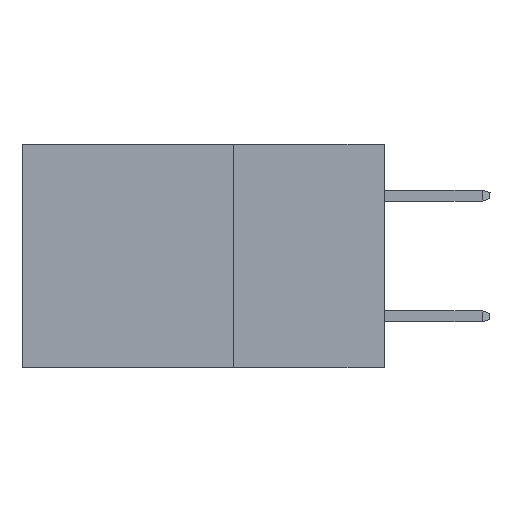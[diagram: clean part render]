
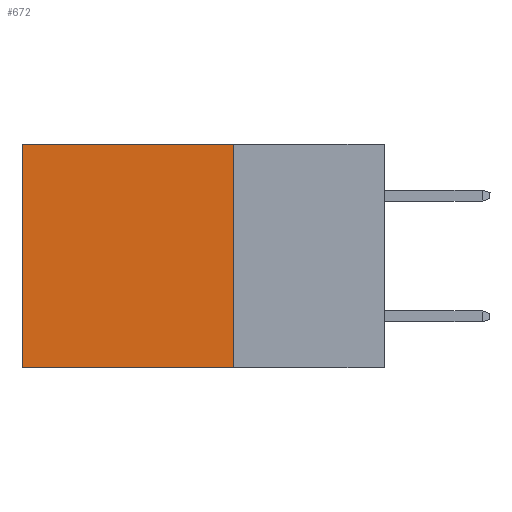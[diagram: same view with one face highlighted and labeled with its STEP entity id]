
A CAD part, left-side view. The second image highlights one B-rep face of the part: STEP entity #672.
In plain terms, the highlighted planar face has unit normal (-1, 0, 0).
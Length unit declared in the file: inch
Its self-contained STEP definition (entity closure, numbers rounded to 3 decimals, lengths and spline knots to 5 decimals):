
#672 = ADVANCED_FACE ( 'NONE', ( #2167 ), #1390, .F. ) ;
#751 = ORIENTED_EDGE ( 'NONE', *, *, #10423, .F. ) ;
#904 = CARTESIAN_POINT ( 'NONE',  ( 0.298, 0.6, 0. ) ) ;
#1065 = CARTESIAN_POINT ( 'NONE',  ( 0.298, 0.6, 0. ) ) ;
#1092 = ORIENTED_EDGE ( 'NONE', *, *, #1553, .F. ) ;
#1360 = LINE ( 'NONE', #7998, #1813 ) ;
#1390 = PLANE ( 'NONE',  #4530 ) ;
#1408 = DIRECTION ( 'NONE',  ( 0., 1., 0. ) ) ;
#1553 = EDGE_CURVE ( 'NONE', #9499, #7437, #1999, .T. ) ;
#1813 = VECTOR ( 'NONE', #3385, 39.37008 ) ;
#1849 = CARTESIAN_POINT ( 'NONE',  ( 0.298, 0.25, 0. ) ) ;
#1999 = LINE ( 'NONE', #6921, #11102 ) ;
#2167 = FACE_OUTER_BOUND ( 'NONE', #8779, .T. ) ;
#2579 = VECTOR ( 'NONE', #4663, 39.37008 ) ;
#3385 = DIRECTION ( 'NONE',  ( 0., 0., -1. ) ) ;
#3850 = LINE ( 'NONE', #904, #8636 ) ;
#4530 = AXIS2_PLACEMENT_3D ( 'NONE', #6015, #6788, #7035 ) ;
#4585 = EDGE_CURVE ( 'NONE', #6712, #10845, #6578, .T. ) ;
#4663 = DIRECTION ( 'NONE',  ( 0., 1., 0. ) ) ;
#5018 = ORIENTED_EDGE ( 'NONE', *, *, #9315, .T. ) ;
#5598 = CARTESIAN_POINT ( 'NONE',  ( 0.298, 0.25, -0.37 ) ) ;
#6015 = CARTESIAN_POINT ( 'NONE',  ( 0.298, 0.25, 0. ) ) ;
#6381 = DIRECTION ( 'NONE',  ( 0., 0., -1. ) ) ;
#6578 = LINE ( 'NONE', #8092, #2579 ) ;
#6712 = VERTEX_POINT ( 'NONE', #1849 ) ;
#6788 = DIRECTION ( 'NONE',  ( 1., 0., 0. ) ) ;
#6921 = CARTESIAN_POINT ( 'NONE',  ( 0.298, 0.25, -0.37 ) ) ;
#7035 = DIRECTION ( 'NONE',  ( 0., 0., -1. ) ) ;
#7437 = VERTEX_POINT ( 'NONE', #8575 ) ;
#7998 = CARTESIAN_POINT ( 'NONE',  ( 0.298, 0.25, 0. ) ) ;
#8092 = CARTESIAN_POINT ( 'NONE',  ( 0.298, 0.25, 0. ) ) ;
#8575 = CARTESIAN_POINT ( 'NONE',  ( 0.298, 0.6, -0.37 ) ) ;
#8636 = VECTOR ( 'NONE', #6381, 39.37008 ) ;
#8779 = EDGE_LOOP ( 'NONE', ( #5018, #1092, #751, #11189 ) ) ;
#9315 = EDGE_CURVE ( 'NONE', #10845, #7437, #3850, .T. ) ;
#9499 = VERTEX_POINT ( 'NONE', #5598 ) ;
#10423 = EDGE_CURVE ( 'NONE', #6712, #9499, #1360, .T. ) ;
#10845 = VERTEX_POINT ( 'NONE', #1065 ) ;
#11102 = VECTOR ( 'NONE', #1408, 39.37008 ) ;
#11189 = ORIENTED_EDGE ( 'NONE', *, *, #4585, .T. ) ;
